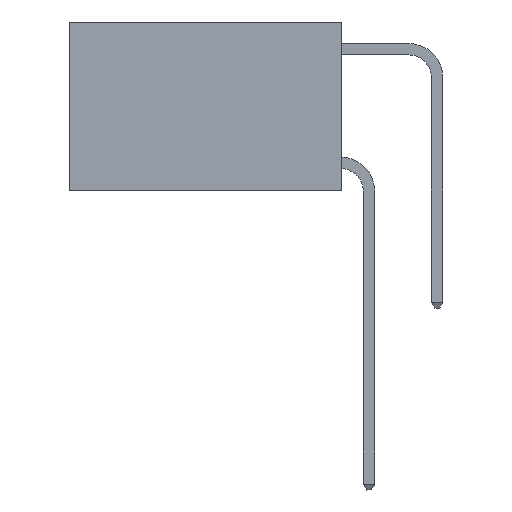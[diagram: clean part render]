
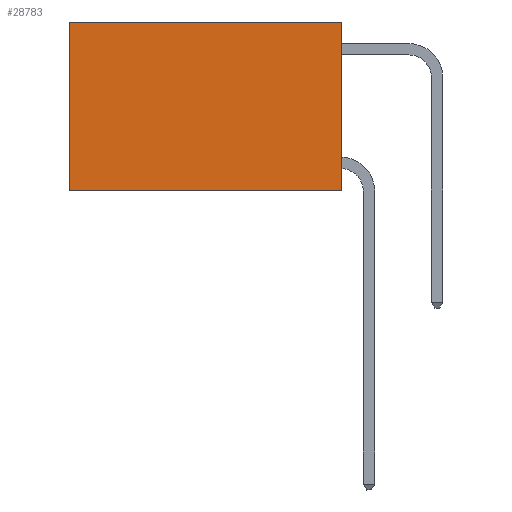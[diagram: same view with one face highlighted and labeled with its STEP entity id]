
A CAD part, left-side view. The second image highlights one B-rep face of the part: STEP entity #28783.
In plain terms, the highlighted planar face has unit normal (-1, 0, 0).
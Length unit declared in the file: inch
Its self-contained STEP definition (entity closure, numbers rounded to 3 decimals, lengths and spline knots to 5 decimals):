
#53 = VECTOR ( 'NONE', #4261, 39.37008 ) ;
#532 = LINE ( 'NONE', #9896, #6543 ) ;
#688 = EDGE_CURVE ( 'NONE', #9139, #16893, #3916, .T. ) ;
#1414 = VECTOR ( 'NONE', #21060, 39.37008 ) ;
#3400 = CARTESIAN_POINT ( 'NONE',  ( 0.2625, 0.6, -0.37 ) ) ;
#3892 = EDGE_CURVE ( 'NONE', #16893, #16496, #532, .T. ) ;
#3916 = LINE ( 'NONE', #14888, #29813 ) ;
#4261 = DIRECTION ( 'NONE',  ( 0., 1., 0. ) ) ;
#4468 = VERTEX_POINT ( 'NONE', #14645 ) ;
#6543 = VECTOR ( 'NONE', #29810, 39.37008 ) ;
#8650 = PLANE ( 'NONE',  #16440 ) ;
#9139 = VERTEX_POINT ( 'NONE', #14681 ) ;
#9896 = CARTESIAN_POINT ( 'NONE',  ( 0.2625, 0., -0.37 ) ) ;
#10107 = EDGE_CURVE ( 'NONE', #4468, #16496, #14968, .T. ) ;
#12552 = ORIENTED_EDGE ( 'NONE', *, *, #21065, .T. ) ;
#13456 = ORIENTED_EDGE ( 'NONE', *, *, #10107, .T. ) ;
#13795 = DIRECTION ( 'NONE',  ( 0., 0., -1. ) ) ;
#14645 = CARTESIAN_POINT ( 'NONE',  ( 0.2625, 0.6, 0. ) ) ;
#14677 = DIRECTION ( 'NONE',  ( 0., 0., -1. ) ) ;
#14681 = CARTESIAN_POINT ( 'NONE',  ( 0.2625, 0., 0. ) ) ;
#14840 = ORIENTED_EDGE ( 'NONE', *, *, #3892, .F. ) ;
#14888 = CARTESIAN_POINT ( 'NONE',  ( 0.2625, 0., 0. ) ) ;
#14968 = LINE ( 'NONE', #16064, #1414 ) ;
#16064 = CARTESIAN_POINT ( 'NONE',  ( 0.2625, 0.6, 0. ) ) ;
#16440 = AXIS2_PLACEMENT_3D ( 'NONE', #26195, #28705, #13795 ) ;
#16496 = VERTEX_POINT ( 'NONE', #3400 ) ;
#16893 = VERTEX_POINT ( 'NONE', #24798 ) ;
#17251 = FACE_OUTER_BOUND ( 'NONE', #23562, .T. ) ;
#20302 = LINE ( 'NONE', #31795, #53 ) ;
#21060 = DIRECTION ( 'NONE',  ( 0., 0., -1. ) ) ;
#21065 = EDGE_CURVE ( 'NONE', #9139, #4468, #20302, .T. ) ;
#23562 = EDGE_LOOP ( 'NONE', ( #13456, #14840, #25621, #12552 ) ) ;
#24798 = CARTESIAN_POINT ( 'NONE',  ( 0.2625, 0., -0.37 ) ) ;
#25621 = ORIENTED_EDGE ( 'NONE', *, *, #688, .F. ) ;
#26195 = CARTESIAN_POINT ( 'NONE',  ( 0.2625, 0., 0. ) ) ;
#28705 = DIRECTION ( 'NONE',  ( 1., 0., 0. ) ) ;
#28783 = ADVANCED_FACE ( 'NONE', ( #17251 ), #8650, .F. ) ;
#29810 = DIRECTION ( 'NONE',  ( 0., 1., 0. ) ) ;
#29813 = VECTOR ( 'NONE', #14677, 39.37008 ) ;
#31795 = CARTESIAN_POINT ( 'NONE',  ( 0.2625, 0., 0. ) ) ;
